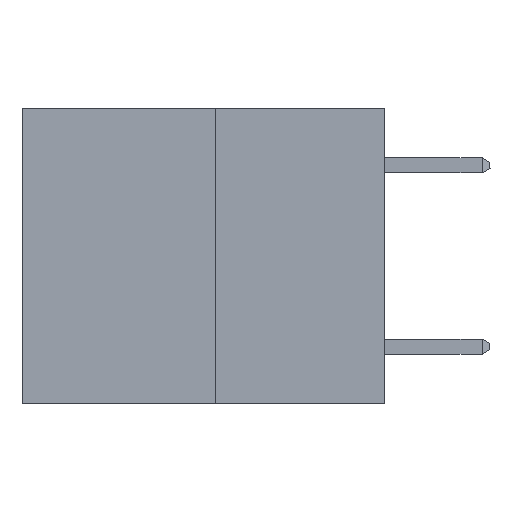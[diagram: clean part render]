
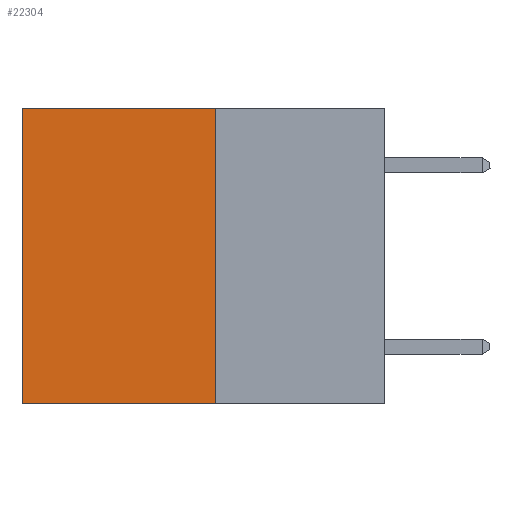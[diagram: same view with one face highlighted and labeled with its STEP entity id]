
A CAD part, left-side view. The second image highlights one B-rep face of the part: STEP entity #22304.
In plain terms, the highlighted planar face has unit normal (-1, 0, 0).
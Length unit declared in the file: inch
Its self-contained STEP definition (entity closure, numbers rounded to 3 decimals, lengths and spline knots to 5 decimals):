
#291 = DIRECTION ( 'NONE',  ( 0., 0., -1. ) ) ;
#656 = VERTEX_POINT ( 'NONE', #15596 ) ;
#1153 = EDGE_CURVE ( 'NONE', #21249, #656, #23000, .T. ) ;
#2169 = EDGE_LOOP ( 'NONE', ( #13946, #9738, #10193, #10980 ) ) ;
#2546 = PLANE ( 'NONE',  #3923 ) ;
#3100 = CARTESIAN_POINT ( 'NONE',  ( 0.3165, 0.28, 0. ) ) ;
#3923 = AXIS2_PLACEMENT_3D ( 'NONE', #10893, #12965, #14973 ) ;
#4274 = VERTEX_POINT ( 'NONE', #21412 ) ;
#4605 = CARTESIAN_POINT ( 'NONE',  ( 0.3165, 0.6, 0. ) ) ;
#5013 = DIRECTION ( 'NONE',  ( 0., 1., 0. ) ) ;
#6997 = LINE ( 'NONE', #13051, #20694 ) ;
#8283 = VECTOR ( 'NONE', #11370, 39.37008 ) ;
#8508 = CARTESIAN_POINT ( 'NONE',  ( 0.3165, 0.6, -0.49 ) ) ;
#9738 = ORIENTED_EDGE ( 'NONE', *, *, #23682, .F. ) ;
#9754 = EDGE_CURVE ( 'NONE', #24422, #21249, #18896, .T. ) ;
#10193 = ORIENTED_EDGE ( 'NONE', *, *, #22642, .F. ) ;
#10859 = FACE_OUTER_BOUND ( 'NONE', #2169, .T. ) ;
#10893 = CARTESIAN_POINT ( 'NONE',  ( 0.3165, 0.28, -0.49 ) ) ;
#10980 = ORIENTED_EDGE ( 'NONE', *, *, #9754, .T. ) ;
#11370 = DIRECTION ( 'NONE',  ( 0., 0., -1. ) ) ;
#12119 = VECTOR ( 'NONE', #291, 39.37008 ) ;
#12424 = LINE ( 'NONE', #21479, #8283 ) ;
#12965 = DIRECTION ( 'NONE',  ( 1., 0., 0. ) ) ;
#13051 = CARTESIAN_POINT ( 'NONE',  ( 0.3165, 0.28, -0.49 ) ) ;
#13946 = ORIENTED_EDGE ( 'NONE', *, *, #1153, .T. ) ;
#14973 = DIRECTION ( 'NONE',  ( 0., 0., -1. ) ) ;
#15596 = CARTESIAN_POINT ( 'NONE',  ( 0.3165, 0.6, -0.49 ) ) ;
#18105 = CARTESIAN_POINT ( 'NONE',  ( 0.3165, 0.28, 0. ) ) ;
#18896 = LINE ( 'NONE', #3100, #23091 ) ;
#20694 = VECTOR ( 'NONE', #5013, 39.37008 ) ;
#21249 = VERTEX_POINT ( 'NONE', #4605 ) ;
#21412 = CARTESIAN_POINT ( 'NONE',  ( 0.3165, 0.28, -0.49 ) ) ;
#21479 = CARTESIAN_POINT ( 'NONE',  ( 0.3165, 0.28, -0.49 ) ) ;
#21800 = DIRECTION ( 'NONE',  ( 0., 1., 0. ) ) ;
#22304 = ADVANCED_FACE ( 'NONE', ( #10859 ), #2546, .F. ) ;
#22642 = EDGE_CURVE ( 'NONE', #24422, #4274, #12424, .T. ) ;
#23000 = LINE ( 'NONE', #8508, #12119 ) ;
#23091 = VECTOR ( 'NONE', #21800, 39.37008 ) ;
#23682 = EDGE_CURVE ( 'NONE', #4274, #656, #6997, .T. ) ;
#24422 = VERTEX_POINT ( 'NONE', #18105 ) ;
